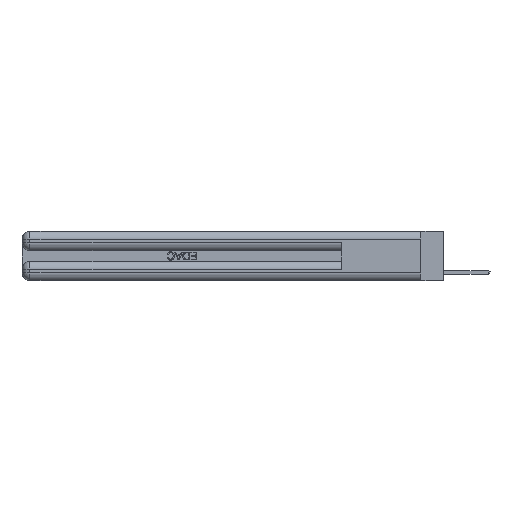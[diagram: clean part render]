
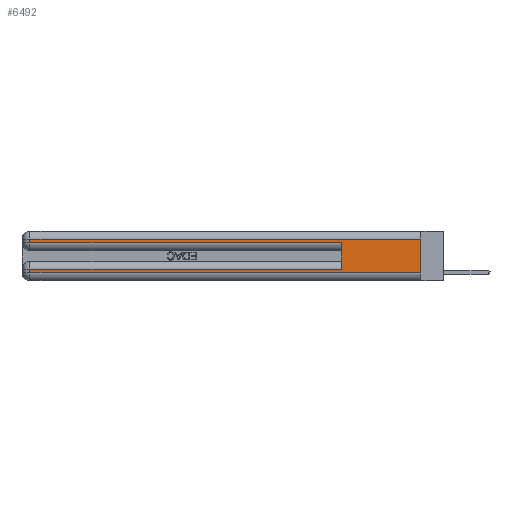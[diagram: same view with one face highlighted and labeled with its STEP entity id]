
A CAD part, left-side view. The second image highlights one B-rep face of the part: STEP entity #6492.
In plain terms, the highlighted planar face has unit normal (-1, 0, 0).
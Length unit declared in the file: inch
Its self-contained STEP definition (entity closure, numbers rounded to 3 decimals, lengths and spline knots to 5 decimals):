
#1084 = CARTESIAN_POINT ( 'NONE',  ( 0., 2.94, 0.31 ) ) ;
#1287 = ORIENTED_EDGE ( 'NONE', *, *, #7014, .T. ) ;
#2683 = PLANE ( 'NONE',  #30070 ) ;
#2925 = CARTESIAN_POINT ( 'NONE',  ( 0., 2.94, 0.06 ) ) ;
#3343 = DIRECTION ( 'NONE',  ( 0., 0., -1. ) ) ;
#3761 = LINE ( 'NONE', #24307, #13867 ) ;
#4306 = DIRECTION ( 'NONE',  ( 0., -1., 0. ) ) ;
#4350 = ORIENTED_EDGE ( 'NONE', *, *, #25265, .T. ) ;
#4580 = VECTOR ( 'NONE', #18236, 39.37008 ) ;
#4668 = VECTOR ( 'NONE', #7922, 39.37008 ) ;
#5179 = VERTEX_POINT ( 'NONE', #23723 ) ;
#5229 = CARTESIAN_POINT ( 'NONE',  ( 0., 2.94, 0.37 ) ) ;
#5891 = VECTOR ( 'NONE', #4306, 39.37008 ) ;
#6469 = DIRECTION ( 'NONE',  ( 0., 0., 1. ) ) ;
#6492 = ADVANCED_FACE ( 'NONE', ( #28629 ), #2683, .F. ) ;
#6711 = VERTEX_POINT ( 'NONE', #32645 ) ;
#7014 = EDGE_CURVE ( 'NONE', #8103, #25801, #14580, .T. ) ;
#7792 = CARTESIAN_POINT ( 'NONE',  ( 0., 0.6, 0.285 ) ) ;
#7881 = DIRECTION ( 'NONE',  ( 1., 0., 0. ) ) ;
#7906 = VECTOR ( 'NONE', #3343, 39.37008 ) ;
#7922 = DIRECTION ( 'NONE',  ( 0., 0., -1. ) ) ;
#8103 = VERTEX_POINT ( 'NONE', #32469 ) ;
#9110 = CARTESIAN_POINT ( 'NONE',  ( 0., 2.94, 0.085 ) ) ;
#9729 = LINE ( 'NONE', #12417, #26293 ) ;
#9997 = ORIENTED_EDGE ( 'NONE', *, *, #19187, .T. ) ;
#10300 = EDGE_CURVE ( 'NONE', #32215, #28571, #15666, .T. ) ;
#10385 = ORIENTED_EDGE ( 'NONE', *, *, #28793, .F. ) ;
#12417 = CARTESIAN_POINT ( 'NONE',  ( 0., 0., 0.06 ) ) ;
#12549 = CARTESIAN_POINT ( 'NONE',  ( 0., 0., 0.285 ) ) ;
#13594 = DIRECTION ( 'NONE',  ( 0., 1., 0. ) ) ;
#13867 = VECTOR ( 'NONE', #6469, 39.37008 ) ;
#14469 = ORIENTED_EDGE ( 'NONE', *, *, #18641, .T. ) ;
#14580 = LINE ( 'NONE', #12549, #5891 ) ;
#14618 = ORIENTED_EDGE ( 'NONE', *, *, #17516, .T. ) ;
#15666 = LINE ( 'NONE', #5229, #4668 ) ;
#15850 = DIRECTION ( 'NONE',  ( 0., 0., -1. ) ) ;
#15892 = EDGE_CURVE ( 'NONE', #27078, #5179, #18255, .T. ) ;
#16013 = CARTESIAN_POINT ( 'NONE',  ( 0., 0., 0.085 ) ) ;
#16145 = LINE ( 'NONE', #26440, #7906 ) ;
#17516 = EDGE_CURVE ( 'NONE', #23355, #8103, #16145, .T. ) ;
#18173 = DIRECTION ( 'NONE',  ( 0., 0., -1. ) ) ;
#18236 = DIRECTION ( 'NONE',  ( 0., 1., 0. ) ) ;
#18255 = LINE ( 'NONE', #28538, #26668 ) ;
#18641 = EDGE_CURVE ( 'NONE', #6711, #32215, #29028, .T. ) ;
#19187 = EDGE_CURVE ( 'NONE', #27078, #23355, #31795, .T. ) ;
#20162 = DIRECTION ( 'NONE',  ( 0., -1., 0. ) ) ;
#20583 = VECTOR ( 'NONE', #13594, 39.37008 ) ;
#23238 = CARTESIAN_POINT ( 'NONE',  ( 0., 0., 0.37 ) ) ;
#23355 = VERTEX_POINT ( 'NONE', #1084 ) ;
#23723 = CARTESIAN_POINT ( 'NONE',  ( 0., 0., 0.06 ) ) ;
#23956 = EDGE_LOOP ( 'NONE', ( #24501, #9997, #14618, #1287, #10385, #14469, #23972, #4350 ) ) ;
#23972 = ORIENTED_EDGE ( 'NONE', *, *, #10300, .T. ) ;
#24307 = CARTESIAN_POINT ( 'NONE',  ( 0., 0.6, 0.145 ) ) ;
#24501 = ORIENTED_EDGE ( 'NONE', *, *, #15892, .F. ) ;
#25265 = EDGE_CURVE ( 'NONE', #28571, #5179, #9729, .T. ) ;
#25801 = VERTEX_POINT ( 'NONE', #7792 ) ;
#26293 = VECTOR ( 'NONE', #20162, 39.37008 ) ;
#26440 = CARTESIAN_POINT ( 'NONE',  ( 0., 2.94, 0.37 ) ) ;
#26668 = VECTOR ( 'NONE', #15850, 39.37008 ) ;
#27078 = VERTEX_POINT ( 'NONE', #30575 ) ;
#28538 = CARTESIAN_POINT ( 'NONE',  ( 0., 0., 0.37 ) ) ;
#28571 = VERTEX_POINT ( 'NONE', #2925 ) ;
#28629 = FACE_OUTER_BOUND ( 'NONE', #23956, .T. ) ;
#28793 = EDGE_CURVE ( 'NONE', #6711, #25801, #3761, .T. ) ;
#29028 = LINE ( 'NONE', #16013, #4580 ) ;
#30070 = AXIS2_PLACEMENT_3D ( 'NONE', #23238, #7881, #18173 ) ;
#30575 = CARTESIAN_POINT ( 'NONE',  ( 0., 0., 0.31 ) ) ;
#31293 = CARTESIAN_POINT ( 'NONE',  ( 0., 0., 0.31 ) ) ;
#31795 = LINE ( 'NONE', #31293, #20583 ) ;
#32215 = VERTEX_POINT ( 'NONE', #9110 ) ;
#32469 = CARTESIAN_POINT ( 'NONE',  ( 0., 2.94, 0.285 ) ) ;
#32645 = CARTESIAN_POINT ( 'NONE',  ( 0., 0.6, 0.085 ) ) ;
